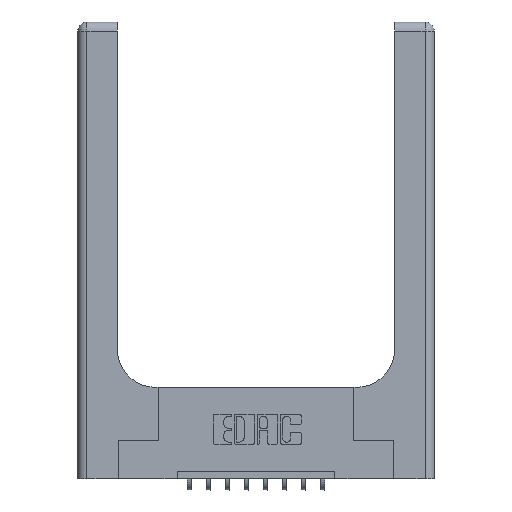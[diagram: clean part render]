
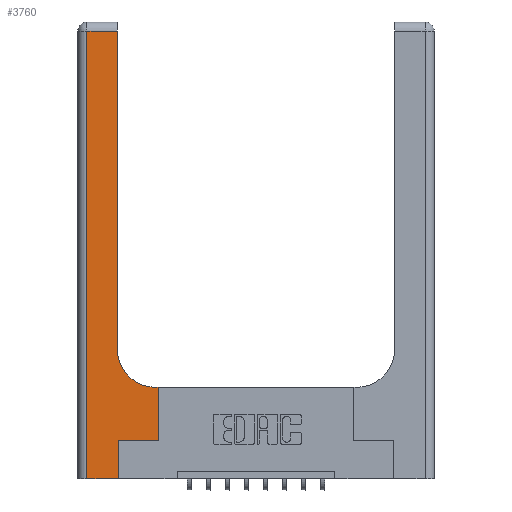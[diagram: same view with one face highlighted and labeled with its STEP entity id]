
A CAD part, top view. The second image highlights one B-rep face of the part: STEP entity #3760.
In plain terms, the highlighted planar face has unit normal (0, 0, 1).
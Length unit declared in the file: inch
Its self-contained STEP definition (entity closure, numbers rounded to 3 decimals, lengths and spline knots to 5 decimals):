
#270 = VECTOR ( 'NONE', #14652, 39.37008 ) ;
#441 = DIRECTION ( 'NONE',  ( 0., 0., -1. ) ) ;
#442 = CARTESIAN_POINT ( 'NONE',  ( 0.265, 0., 0.37 ) ) ;
#462 = LINE ( 'NONE', #11967, #5659 ) ;
#498 = CARTESIAN_POINT ( 'NONE',  ( 0.528, 0.6, 0.37 ) ) ;
#509 = FACE_OUTER_BOUND ( 'NONE', #10955, .T. ) ;
#741 = VERTEX_POINT ( 'NONE', #6057 ) ;
#806 = VECTOR ( 'NONE', #1985, 39.37008 ) ;
#982 = DIRECTION ( 'NONE',  ( 1., 0., 0. ) ) ;
#1010 = VERTEX_POINT ( 'NONE', #13271 ) ;
#1788 = EDGE_CURVE ( 'NONE', #14306, #3672, #3367, .T. ) ;
#1985 = DIRECTION ( 'NONE',  ( 0., -1., 0. ) ) ;
#1998 = VECTOR ( 'NONE', #13198, 39.37008 ) ;
#2129 = DIRECTION ( 'NONE',  ( 1., 0., 0. ) ) ;
#2147 = LINE ( 'NONE', #6995, #2160 ) ;
#2160 = VECTOR ( 'NONE', #11752, 39.37008 ) ;
#2165 = LINE ( 'NONE', #9184, #270 ) ;
#2352 = DIRECTION ( 'NONE',  ( 0., 0., -1. ) ) ;
#2564 = VECTOR ( 'NONE', #6916, 39.37008 ) ;
#3062 = CARTESIAN_POINT ( 'NONE',  ( 0.528, 0.25, 0.37 ) ) ;
#3367 = LINE ( 'NONE', #12833, #2564 ) ;
#3672 = VERTEX_POINT ( 'NONE', #13742 ) ;
#3760 = ADVANCED_FACE ( 'NONE', ( #509 ), #4879, .F. ) ;
#4819 = LINE ( 'NONE', #8001, #13368 ) ;
#4879 = PLANE ( 'NONE',  #6977 ) ;
#4897 = DIRECTION ( 'NONE',  ( -1., 0., 0. ) ) ;
#5147 = ORIENTED_EDGE ( 'NONE', *, *, #13011, .T. ) ;
#5180 = CARTESIAN_POINT ( 'NONE',  ( 0., 3., 0.37 ) ) ;
#5288 = CARTESIAN_POINT ( 'NONE',  ( 0.26, 0.85, 0.37 ) ) ;
#5432 = EDGE_CURVE ( 'NONE', #3672, #741, #2147, .T. ) ;
#5659 = VECTOR ( 'NONE', #4897, 39.37008 ) ;
#6057 = CARTESIAN_POINT ( 'NONE',  ( 0.06, 2.94, 0.37 ) ) ;
#6166 = AXIS2_PLACEMENT_3D ( 'NONE', #11579, #2352, #2129 ) ;
#6285 = ORIENTED_EDGE ( 'NONE', *, *, #11471, .T. ) ;
#6769 = CARTESIAN_POINT ( 'NONE',  ( 0.06, 3., 0.37 ) ) ;
#6916 = DIRECTION ( 'NONE',  ( 0., 1., 0. ) ) ;
#6977 = AXIS2_PLACEMENT_3D ( 'NONE', #5180, #441, #13272 ) ;
#6995 = CARTESIAN_POINT ( 'NONE',  ( 0., 2.94, 0.37 ) ) ;
#7006 = VERTEX_POINT ( 'NONE', #9791 ) ;
#7836 = ORIENTED_EDGE ( 'NONE', *, *, #5432, .T. ) ;
#7933 = LINE ( 'NONE', #6769, #806 ) ;
#8001 = CARTESIAN_POINT ( 'NONE',  ( 0., 0., 0.37 ) ) ;
#8214 = CARTESIAN_POINT ( 'NONE',  ( 0.528, 0.25, 0.37 ) ) ;
#8289 = LINE ( 'NONE', #8214, #13909 ) ;
#8341 = ORIENTED_EDGE ( 'NONE', *, *, #14378, .T. ) ;
#8435 = LINE ( 'NONE', #8662, #1998 ) ;
#8662 = CARTESIAN_POINT ( 'NONE',  ( 0.265, 0.25, 0.37 ) ) ;
#9184 = CARTESIAN_POINT ( 'NONE',  ( 0.265, 0., 0.37 ) ) ;
#9418 = EDGE_CURVE ( 'NONE', #11953, #7006, #2165, .T. ) ;
#9767 = ORIENTED_EDGE ( 'NONE', *, *, #9418, .T. ) ;
#9791 = CARTESIAN_POINT ( 'NONE',  ( 0.265, 0.25, 0.37 ) ) ;
#10119 = CIRCLE ( 'NONE', #6166, 0.25 ) ;
#10416 = EDGE_CURVE ( 'NONE', #14354, #14306, #10119, .T. ) ;
#10686 = CARTESIAN_POINT ( 'NONE',  ( 0.51, 0.6, 0.37 ) ) ;
#10955 = EDGE_LOOP ( 'NONE', ( #13059, #7836, #5147, #12531, #9767, #12234, #8341, #6285, #14051 ) ) ;
#11221 = VERTEX_POINT ( 'NONE', #3062 ) ;
#11366 = EDGE_CURVE ( 'NONE', #1010, #11953, #4819, .T. ) ;
#11471 = EDGE_CURVE ( 'NONE', #13533, #14354, #462, .T. ) ;
#11579 = CARTESIAN_POINT ( 'NONE',  ( 0.51, 0.85, 0.37 ) ) ;
#11752 = DIRECTION ( 'NONE',  ( -1., 0., 0. ) ) ;
#11953 = VERTEX_POINT ( 'NONE', #442 ) ;
#11965 = EDGE_CURVE ( 'NONE', #7006, #11221, #8435, .T. ) ;
#11967 = CARTESIAN_POINT ( 'NONE',  ( 0.26, 0.6, 0.37 ) ) ;
#12234 = ORIENTED_EDGE ( 'NONE', *, *, #11965, .T. ) ;
#12531 = ORIENTED_EDGE ( 'NONE', *, *, #11366, .T. ) ;
#12833 = CARTESIAN_POINT ( 'NONE',  ( 0.26, 3., 0.37 ) ) ;
#13011 = EDGE_CURVE ( 'NONE', #741, #1010, #7933, .T. ) ;
#13059 = ORIENTED_EDGE ( 'NONE', *, *, #1788, .T. ) ;
#13198 = DIRECTION ( 'NONE',  ( 1., 0., 0. ) ) ;
#13271 = CARTESIAN_POINT ( 'NONE',  ( 0.06, 0., 0.37 ) ) ;
#13272 = DIRECTION ( 'NONE',  ( -1., 0., 0. ) ) ;
#13368 = VECTOR ( 'NONE', #982, 39.37008 ) ;
#13533 = VERTEX_POINT ( 'NONE', #498 ) ;
#13742 = CARTESIAN_POINT ( 'NONE',  ( 0.26, 2.94, 0.37 ) ) ;
#13909 = VECTOR ( 'NONE', #14106, 39.37008 ) ;
#14051 = ORIENTED_EDGE ( 'NONE', *, *, #10416, .T. ) ;
#14106 = DIRECTION ( 'NONE',  ( 0., 1., 0. ) ) ;
#14306 = VERTEX_POINT ( 'NONE', #5288 ) ;
#14354 = VERTEX_POINT ( 'NONE', #10686 ) ;
#14378 = EDGE_CURVE ( 'NONE', #11221, #13533, #8289, .T. ) ;
#14652 = DIRECTION ( 'NONE',  ( 0., 1., 0. ) ) ;
